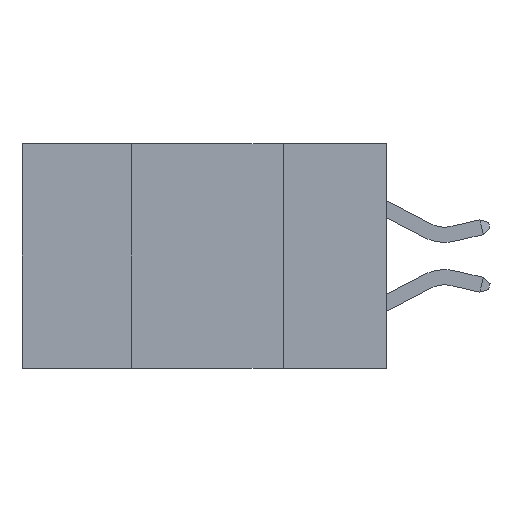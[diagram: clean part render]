
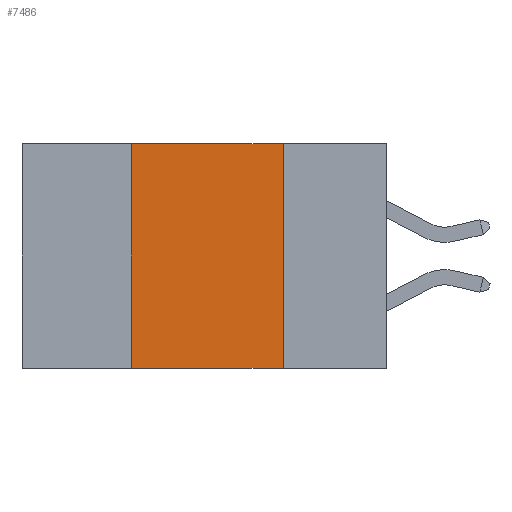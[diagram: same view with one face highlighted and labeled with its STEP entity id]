
A CAD part, left-side view. The second image highlights one B-rep face of the part: STEP entity #7486.
In plain terms, the highlighted planar face has unit normal (-1, 0, 0).
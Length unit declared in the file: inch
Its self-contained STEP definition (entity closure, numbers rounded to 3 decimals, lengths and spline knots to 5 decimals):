
#34 = AXIS2_PLACEMENT_3D ( 'NONE', #2733, #4457, #1130 ) ;
#300 = VERTEX_POINT ( 'NONE', #10426 ) ;
#311 = EDGE_CURVE ( 'NONE', #10496, #726, #2289, .T. ) ;
#726 = VERTEX_POINT ( 'NONE', #2851 ) ;
#1130 = DIRECTION ( 'NONE',  ( 0., 0., -1. ) ) ;
#2289 = LINE ( 'NONE', #9233, #6251 ) ;
#2668 = LINE ( 'NONE', #10606, #4404 ) ;
#2733 = CARTESIAN_POINT ( 'NONE',  ( 0., 0.6, 0. ) ) ;
#2851 = CARTESIAN_POINT ( 'NONE',  ( 0., 0.42, 0. ) ) ;
#3210 = LINE ( 'NONE', #9976, #5189 ) ;
#4401 = VERTEX_POINT ( 'NONE', #8324 ) ;
#4404 = VECTOR ( 'NONE', #8978, 39.37008 ) ;
#4457 = DIRECTION ( 'NONE',  ( 1., 0., 0. ) ) ;
#4914 = ORIENTED_EDGE ( 'NONE', *, *, #311, .F. ) ;
#5189 = VECTOR ( 'NONE', #10850, 39.37008 ) ;
#5350 = EDGE_CURVE ( 'NONE', #4401, #300, #8755, .T. ) ;
#5409 = FACE_OUTER_BOUND ( 'NONE', #6520, .T. ) ;
#5530 = EDGE_CURVE ( 'NONE', #10496, #300, #2668, .T. ) ;
#5929 = EDGE_CURVE ( 'NONE', #726, #4401, #3210, .T. ) ;
#6251 = VECTOR ( 'NONE', #7460, 39.37008 ) ;
#6520 = EDGE_LOOP ( 'NONE', ( #9428, #10636, #4914, #10404 ) ) ;
#6832 = DIRECTION ( 'NONE',  ( 0., 0., -1. ) ) ;
#6940 = CARTESIAN_POINT ( 'NONE',  ( 0., 0.17, 0. ) ) ;
#7460 = DIRECTION ( 'NONE',  ( 0., 0., 1. ) ) ;
#7486 = ADVANCED_FACE ( 'NONE', ( #5409 ), #7882, .F. ) ;
#7882 = PLANE ( 'NONE',  #34 ) ;
#8324 = CARTESIAN_POINT ( 'NONE',  ( 0., 0.17, 0. ) ) ;
#8755 = LINE ( 'NONE', #6940, #10715 ) ;
#8978 = DIRECTION ( 'NONE',  ( 0., -1., 0. ) ) ;
#9233 = CARTESIAN_POINT ( 'NONE',  ( 0., 0.42, 0. ) ) ;
#9428 = ORIENTED_EDGE ( 'NONE', *, *, #5350, .F. ) ;
#9976 = CARTESIAN_POINT ( 'NONE',  ( 0., 0.6, 0. ) ) ;
#10093 = CARTESIAN_POINT ( 'NONE',  ( 0., 0.42, -0.37 ) ) ;
#10404 = ORIENTED_EDGE ( 'NONE', *, *, #5530, .T. ) ;
#10426 = CARTESIAN_POINT ( 'NONE',  ( 0., 0.17, -0.37 ) ) ;
#10496 = VERTEX_POINT ( 'NONE', #10093 ) ;
#10606 = CARTESIAN_POINT ( 'NONE',  ( 0., 0.6, -0.37 ) ) ;
#10636 = ORIENTED_EDGE ( 'NONE', *, *, #5929, .F. ) ;
#10715 = VECTOR ( 'NONE', #6832, 39.37008 ) ;
#10850 = DIRECTION ( 'NONE',  ( 0., -1., 0. ) ) ;
